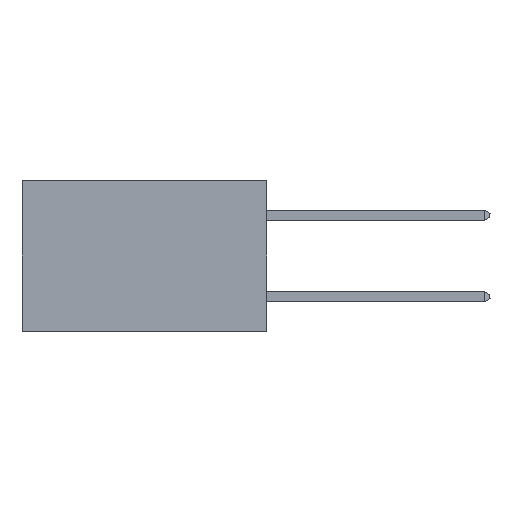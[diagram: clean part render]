
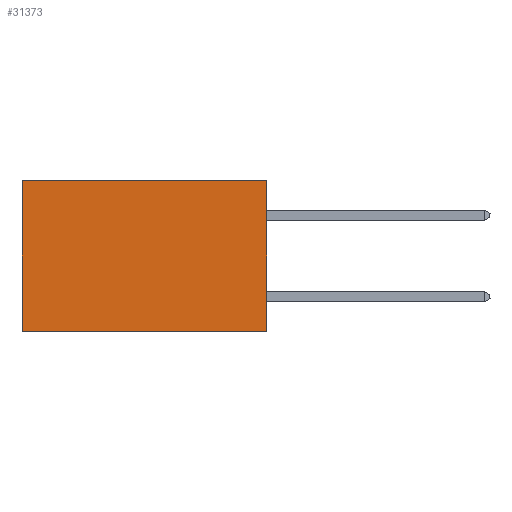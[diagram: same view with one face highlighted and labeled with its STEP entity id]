
A CAD part, left-side view. The second image highlights one B-rep face of the part: STEP entity #31373.
In plain terms, the highlighted planar face has unit normal (-1, 0, 0).
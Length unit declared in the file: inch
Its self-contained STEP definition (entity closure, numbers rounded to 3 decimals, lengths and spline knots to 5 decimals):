
#535 = DIRECTION ( 'NONE',  ( 1., 0., 0. ) ) ;
#1750 = CARTESIAN_POINT ( 'NONE',  ( 0.2875, 0., 0. ) ) ;
#2098 = CARTESIAN_POINT ( 'NONE',  ( 0.2875, 0.6, -0.37 ) ) ;
#4101 = DIRECTION ( 'NONE',  ( 0., 1., 0. ) ) ;
#6021 = ORIENTED_EDGE ( 'NONE', *, *, #17594, .T. ) ;
#7563 = CARTESIAN_POINT ( 'NONE',  ( 0.2875, 0., -0.37 ) ) ;
#8057 = CARTESIAN_POINT ( 'NONE',  ( 0.2875, 0., 0. ) ) ;
#8245 = CARTESIAN_POINT ( 'NONE',  ( 0.2875, 0.6, 0. ) ) ;
#8648 = CARTESIAN_POINT ( 'NONE',  ( 0.2875, 0., 0. ) ) ;
#11124 = VERTEX_POINT ( 'NONE', #43510 ) ;
#15773 = ORIENTED_EDGE ( 'NONE', *, *, #16222, .F. ) ;
#16222 = EDGE_CURVE ( 'NONE', #11124, #22086, #24993, .T. ) ;
#16275 = ORIENTED_EDGE ( 'NONE', *, *, #36574, .F. ) ;
#16576 = VECTOR ( 'NONE', #4101, 39.37008 ) ;
#17594 = EDGE_CURVE ( 'NONE', #17669, #22086, #26588, .T. ) ;
#17669 = VERTEX_POINT ( 'NONE', #8245 ) ;
#19313 = EDGE_CURVE ( 'NONE', #34978, #17669, #23830, .T. ) ;
#20101 = DIRECTION ( 'NONE',  ( 0., 1., 0. ) ) ;
#21824 = DIRECTION ( 'NONE',  ( 0., 0., -1. ) ) ;
#22086 = VERTEX_POINT ( 'NONE', #2098 ) ;
#22824 = CARTESIAN_POINT ( 'NONE',  ( 0.2875, 0.6, 0. ) ) ;
#23789 = FACE_OUTER_BOUND ( 'NONE', #23916, .T. ) ;
#23830 = LINE ( 'NONE', #8648, #43373 ) ;
#23916 = EDGE_LOOP ( 'NONE', ( #6021, #15773, #16275, #46323 ) ) ;
#24486 = AXIS2_PLACEMENT_3D ( 'NONE', #8057, #535, #40445 ) ;
#24993 = LINE ( 'NONE', #7563, #16576 ) ;
#26588 = LINE ( 'NONE', #22824, #27705 ) ;
#27705 = VECTOR ( 'NONE', #33216, 39.37008 ) ;
#28391 = LINE ( 'NONE', #39962, #37314 ) ;
#31373 = ADVANCED_FACE ( 'NONE', ( #23789 ), #36747, .F. ) ;
#33216 = DIRECTION ( 'NONE',  ( 0., 0., -1. ) ) ;
#34978 = VERTEX_POINT ( 'NONE', #1750 ) ;
#36574 = EDGE_CURVE ( 'NONE', #34978, #11124, #28391, .T. ) ;
#36747 = PLANE ( 'NONE',  #24486 ) ;
#37314 = VECTOR ( 'NONE', #21824, 39.37008 ) ;
#39962 = CARTESIAN_POINT ( 'NONE',  ( 0.2875, 0., 0. ) ) ;
#40445 = DIRECTION ( 'NONE',  ( 0., 0., -1. ) ) ;
#43373 = VECTOR ( 'NONE', #20101, 39.37008 ) ;
#43510 = CARTESIAN_POINT ( 'NONE',  ( 0.2875, 0., -0.37 ) ) ;
#46323 = ORIENTED_EDGE ( 'NONE', *, *, #19313, .T. ) ;
